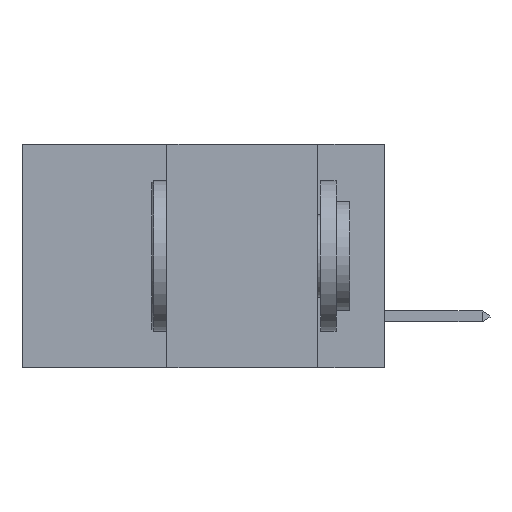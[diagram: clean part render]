
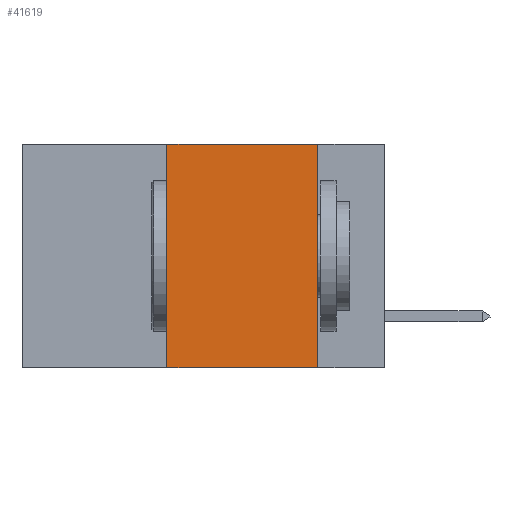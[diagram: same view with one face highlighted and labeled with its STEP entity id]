
A CAD part, left-side view. The second image highlights one B-rep face of the part: STEP entity #41619.
In plain terms, the highlighted planar face has unit normal (-1, 0, 0).
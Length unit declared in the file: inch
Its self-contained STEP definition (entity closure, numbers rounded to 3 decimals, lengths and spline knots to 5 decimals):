
#238 = EDGE_CURVE ( 'NONE', #6984, #28484, #26669, .T. ) ;
#290 = ORIENTED_EDGE ( 'NONE', *, *, #11387, .F. ) ;
#5261 = DIRECTION ( 'NONE',  ( 0., 0., 1. ) ) ;
#5427 = EDGE_CURVE ( 'NONE', #7177, #27799, #14201, .T. ) ;
#6984 = VERTEX_POINT ( 'NONE', #33594 ) ;
#7177 = VERTEX_POINT ( 'NONE', #37542 ) ;
#7670 = CARTESIAN_POINT ( 'NONE',  ( 0., 0.11, -0.37 ) ) ;
#9470 = AXIS2_PLACEMENT_3D ( 'NONE', #32793, #19410, #35877 ) ;
#10320 = EDGE_LOOP ( 'NONE', ( #290, #41548, #20682, #15079 ) ) ;
#10918 = CARTESIAN_POINT ( 'NONE',  ( 0., 0.6, -0.37 ) ) ;
#11344 = CARTESIAN_POINT ( 'NONE',  ( 0., 0.11, 0. ) ) ;
#11387 = EDGE_CURVE ( 'NONE', #27799, #28484, #29454, .T. ) ;
#14201 = LINE ( 'NONE', #26392, #33398 ) ;
#15079 = ORIENTED_EDGE ( 'NONE', *, *, #238, .T. ) ;
#18463 = CARTESIAN_POINT ( 'NONE',  ( 0., 0.11, 0. ) ) ;
#19282 = PLANE ( 'NONE',  #9470 ) ;
#19410 = DIRECTION ( 'NONE',  ( 1., 0., 0. ) ) ;
#20682 = ORIENTED_EDGE ( 'NONE', *, *, #35452, .F. ) ;
#22528 = VECTOR ( 'NONE', #33813, 39.37008 ) ;
#26392 = CARTESIAN_POINT ( 'NONE',  ( 0., 0.6, 0. ) ) ;
#26669 = LINE ( 'NONE', #10918, #22528 ) ;
#27799 = VERTEX_POINT ( 'NONE', #11344 ) ;
#28484 = VERTEX_POINT ( 'NONE', #7670 ) ;
#29454 = LINE ( 'NONE', #18463, #32035 ) ;
#32035 = VECTOR ( 'NONE', #41767, 39.37008 ) ;
#32382 = FACE_OUTER_BOUND ( 'NONE', #10320, .T. ) ;
#32793 = CARTESIAN_POINT ( 'NONE',  ( 0., 0.6, 0. ) ) ;
#33398 = VECTOR ( 'NONE', #42838, 39.37008 ) ;
#33594 = CARTESIAN_POINT ( 'NONE',  ( 0., 0.36, -0.37 ) ) ;
#33813 = DIRECTION ( 'NONE',  ( 0., -1., 0. ) ) ;
#35452 = EDGE_CURVE ( 'NONE', #6984, #7177, #38535, .T. ) ;
#35877 = DIRECTION ( 'NONE',  ( 0., 0., -1. ) ) ;
#37542 = CARTESIAN_POINT ( 'NONE',  ( 0., 0.36, 0. ) ) ;
#38535 = LINE ( 'NONE', #41663, #42179 ) ;
#41548 = ORIENTED_EDGE ( 'NONE', *, *, #5427, .F. ) ;
#41619 = ADVANCED_FACE ( 'NONE', ( #32382 ), #19282, .F. ) ;
#41663 = CARTESIAN_POINT ( 'NONE',  ( 0., 0.36, 0. ) ) ;
#41767 = DIRECTION ( 'NONE',  ( 0., 0., -1. ) ) ;
#42179 = VECTOR ( 'NONE', #5261, 39.37008 ) ;
#42838 = DIRECTION ( 'NONE',  ( 0., -1., 0. ) ) ;
